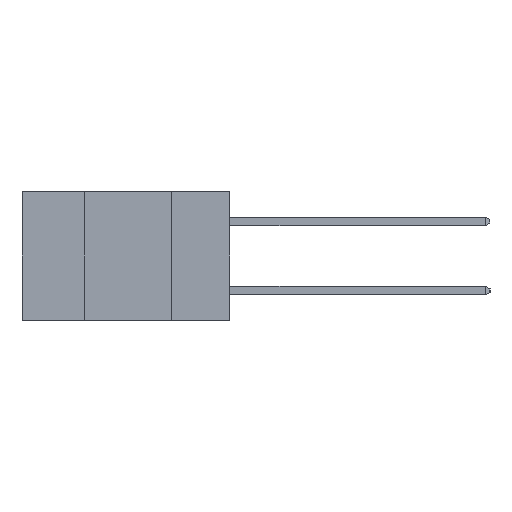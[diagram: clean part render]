
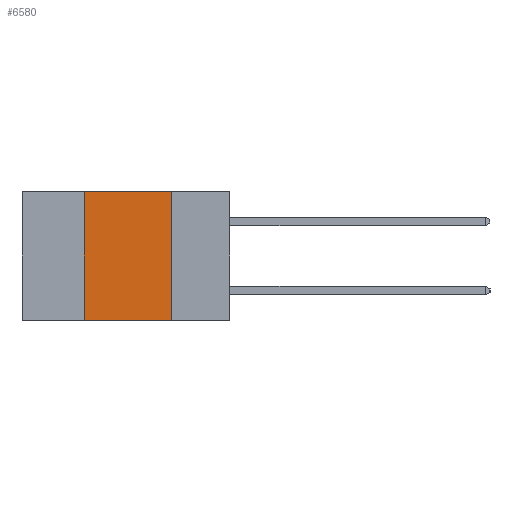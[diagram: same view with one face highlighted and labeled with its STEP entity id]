
A CAD part, left-side view. The second image highlights one B-rep face of the part: STEP entity #6580.
In plain terms, the highlighted planar face has unit normal (-1, 0, 0).
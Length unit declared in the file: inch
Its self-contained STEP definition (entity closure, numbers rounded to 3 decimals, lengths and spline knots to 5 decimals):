
#77 = CARTESIAN_POINT ( 'NONE',  ( 0., 0.17, -0.37 ) ) ;
#206 = DIRECTION ( 'NONE',  ( 0., -1., 0. ) ) ;
#945 = CARTESIAN_POINT ( 'NONE',  ( 0., 0.6, 0. ) ) ;
#1016 = DIRECTION ( 'NONE',  ( 0., 0., 1. ) ) ;
#1153 = VERTEX_POINT ( 'NONE', #3709 ) ;
#2456 = DIRECTION ( 'NONE',  ( 1., 0., 0. ) ) ;
#2810 = VECTOR ( 'NONE', #1016, 39.37008 ) ;
#2813 = AXIS2_PLACEMENT_3D ( 'NONE', #10969, #2456, #12298 ) ;
#3225 = ORIENTED_EDGE ( 'NONE', *, *, #4145, .T. ) ;
#3303 = VECTOR ( 'NONE', #4472, 39.37008 ) ;
#3709 = CARTESIAN_POINT ( 'NONE',  ( 0., 0.42, 0. ) ) ;
#4145 = EDGE_CURVE ( 'NONE', #10304, #5377, #10782, .T. ) ;
#4169 = EDGE_CURVE ( 'NONE', #10304, #1153, #6747, .T. ) ;
#4172 = EDGE_CURVE ( 'NONE', #1153, #14362, #13469, .T. ) ;
#4194 = EDGE_CURVE ( 'NONE', #14362, #5377, #9511, .T. ) ;
#4426 = CARTESIAN_POINT ( 'NONE',  ( 0., 0.17, 0. ) ) ;
#4472 = DIRECTION ( 'NONE',  ( 0., -1., 0. ) ) ;
#4745 = CARTESIAN_POINT ( 'NONE',  ( 0., 0.42, -0.37 ) ) ;
#5020 = CARTESIAN_POINT ( 'NONE',  ( 0., 0.6, -0.37 ) ) ;
#5377 = VERTEX_POINT ( 'NONE', #7682 ) ;
#5861 = VECTOR ( 'NONE', #13110, 39.37008 ) ;
#6298 = VECTOR ( 'NONE', #206, 39.37008 ) ;
#6580 = ADVANCED_FACE ( 'NONE', ( #12616 ), #14943, .F. ) ;
#6747 = LINE ( 'NONE', #4745, #2810 ) ;
#7545 = ORIENTED_EDGE ( 'NONE', *, *, #4172, .F. ) ;
#7682 = CARTESIAN_POINT ( 'NONE',  ( 0., 0.17, -0.37 ) ) ;
#8980 = EDGE_LOOP ( 'NONE', ( #11142, #7545, #10720, #3225 ) ) ;
#9511 = LINE ( 'NONE', #77, #5861 ) ;
#10304 = VERTEX_POINT ( 'NONE', #14819 ) ;
#10720 = ORIENTED_EDGE ( 'NONE', *, *, #4169, .F. ) ;
#10782 = LINE ( 'NONE', #5020, #3303 ) ;
#10969 = CARTESIAN_POINT ( 'NONE',  ( 0., 0.6, 0. ) ) ;
#11142 = ORIENTED_EDGE ( 'NONE', *, *, #4194, .F. ) ;
#12298 = DIRECTION ( 'NONE',  ( 0., 0., -1. ) ) ;
#12616 = FACE_OUTER_BOUND ( 'NONE', #8980, .T. ) ;
#13110 = DIRECTION ( 'NONE',  ( 0., 0., -1. ) ) ;
#13469 = LINE ( 'NONE', #945, #6298 ) ;
#14362 = VERTEX_POINT ( 'NONE', #4426 ) ;
#14819 = CARTESIAN_POINT ( 'NONE',  ( 0., 0.42, -0.37 ) ) ;
#14943 = PLANE ( 'NONE',  #2813 ) ;
